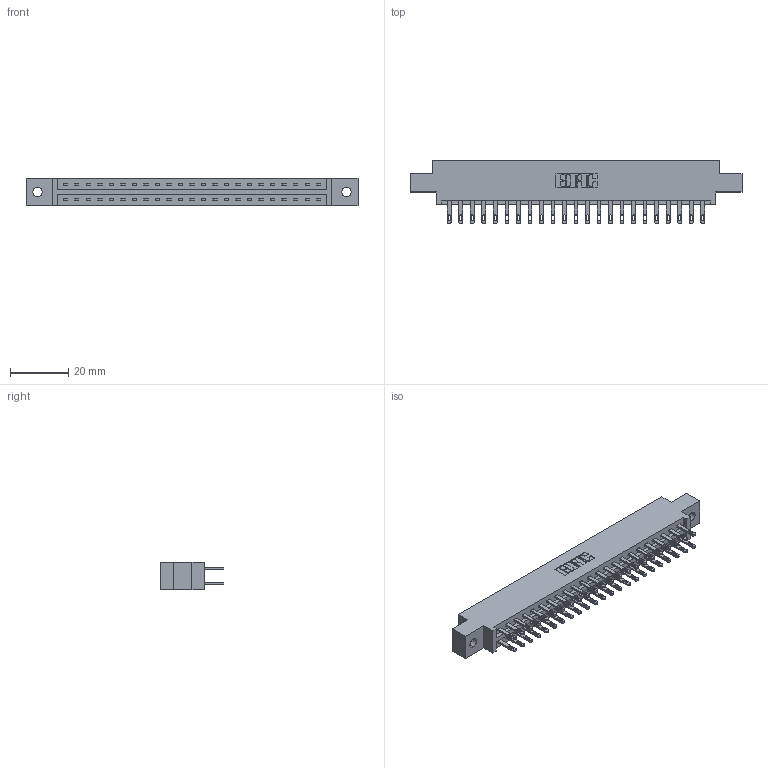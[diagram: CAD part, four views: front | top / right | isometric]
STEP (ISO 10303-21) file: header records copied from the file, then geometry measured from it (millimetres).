
FILE_DESCRIPTION (( 'STEP AP203' ), '1' );
FILE_NAME ('337-046-500-802.STEP', '2019-10-11T14:09:00', ( '' ), ( '' ), 'SwSTEP 2.0', 'SolidWorks 2016', '' );
FILE_SCHEMA (( 'CONFIG_CONTROL_DESIGN' ));
Length unit declared in the file: inch
Products named in the file (3): 337-046-500-802; 337 Part_0.170 Offset - 0.128 Dia; 345-292-001_345-293-100
Assembly tree (47 placements, depth 2):
  337-046-500-802
    337 Part_0.170 Offset - 0.128 Dia
    345-292-001_345-293-100  x46
Bounding box: 114.15 x 21.85 x 9.4 mm (x, y, z)
Volume: 11763.2 mm3; surface area: 13459.3 mm2
Topology: 47 solids, 47 shells, 2418 faces, 7361 edges, 4906 vertices
Faces by surface type: plane 1546, cylinder 872
Entity records: 20355 total; most frequent: CARTESIAN_POINT 3446, ORIENTED_EDGE 3382, DIRECTION 2967, EDGE_CURVE 1691, LINE 1559, VECTOR 1559, VERTEX_POINT 1126, AXIS2_PLACEMENT_3D 704
